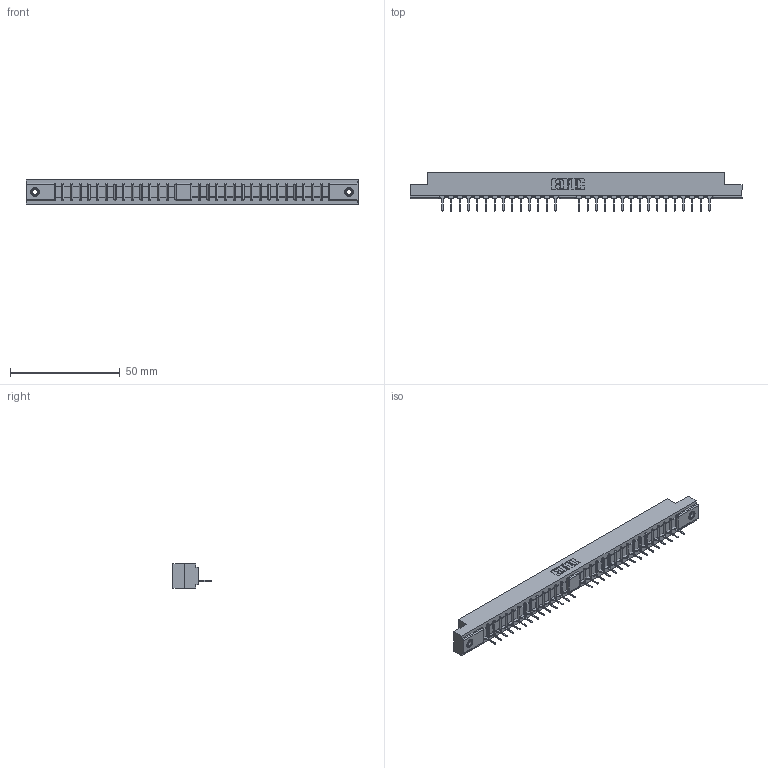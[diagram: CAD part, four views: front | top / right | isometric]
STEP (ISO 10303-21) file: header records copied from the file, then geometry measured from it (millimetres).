
FILE_DESCRIPTION (( 'STEP AP203' ), '1' );
FILE_NAME ('310-030-531-108.STEP', '2020-03-25T12:15:59', ( '' ), ( '' ), 'SwSTEP 2.0', 'SolidWorks 2016', '' );
FILE_SCHEMA (( 'CONFIG_CONTROL_DESIGN' ));
Length unit declared in the file: millimetre
Products named in the file (4): 310 Part_.116 Hex; 310-030-531-108; 345-250-001_345-250-003-102; 307-290-001_531
Assembly tree (33 placements, depth 2):
  310-030-531-108
    310 Part_.116 Hex
    307-290-001_531  x30
    345-250-001_345-250-003-102  x2
Bounding box: 151.21 x 17.37 x 10.97 mm (x, y, z)
Volume: 12607.2 mm3; surface area: 14662.8 mm2
Topology: 33 solids, 33 shells, 1906 faces, 5357 edges, 3434 vertices
Faces by surface type: plane 1226, cylinder 600, sphere 64, cone 12, torus 4
Entity records: 28775 total; most frequent: CARTESIAN_POINT 4824, ORIENTED_EDGE 4802, DIRECTION 4709, EDGE_CURVE 2401, VECTOR 1843, LINE 1843, VERTEX_POINT 1548, AXIS2_PLACEMENT_3D 1433
